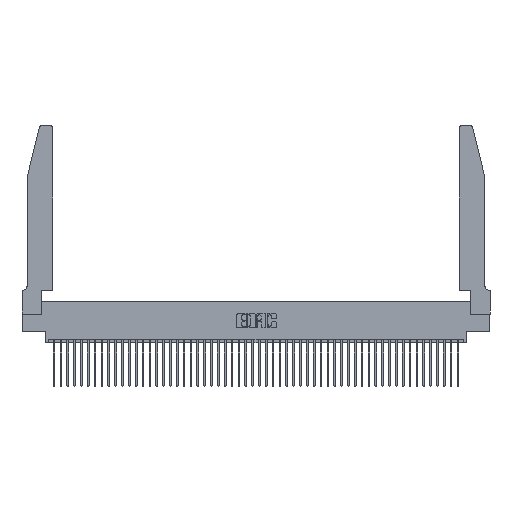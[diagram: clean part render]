
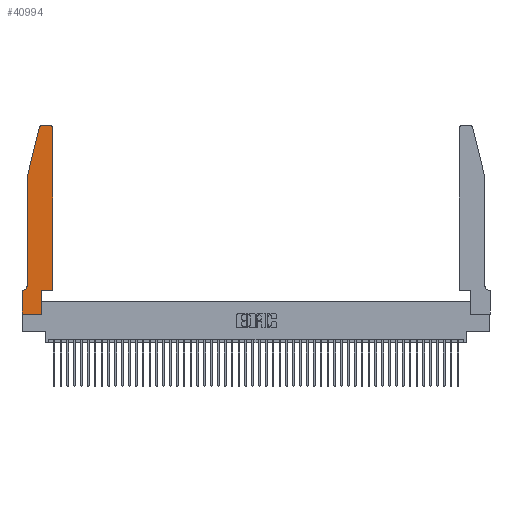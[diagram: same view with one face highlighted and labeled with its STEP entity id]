
A CAD part, top view. The second image highlights one B-rep face of the part: STEP entity #40994.
In plain terms, the highlighted planar face has unit normal (0, 0, 1).
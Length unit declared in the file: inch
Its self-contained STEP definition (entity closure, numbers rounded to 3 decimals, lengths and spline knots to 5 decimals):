
#375 = VERTEX_POINT ( 'NONE', #23162 ) ;
#771 = VERTEX_POINT ( 'NONE', #3307 ) ;
#784 = DIRECTION ( 'NONE',  ( 1., 0., 0. ) ) ;
#2011 = LINE ( 'NONE', #36926, #9230 ) ;
#2113 = VECTOR ( 'NONE', #45506, 39.37008 ) ;
#2149 = EDGE_CURVE ( 'NONE', #18100, #37735, #42309, .T. ) ;
#2790 = DIRECTION ( 'NONE',  ( 0., 0., 1. ) ) ;
#2897 = EDGE_CURVE ( 'NONE', #375, #42579, #21915, .T. ) ;
#3307 = CARTESIAN_POINT ( 'NONE',  ( 0.4505, 0.35, 0.37 ) ) ;
#3364 = ORIENTED_EDGE ( 'NONE', *, *, #41701, .T. ) ;
#5759 = EDGE_CURVE ( 'NONE', #32622, #375, #25288, .T. ) ;
#6160 = VECTOR ( 'NONE', #47278, 39.37008 ) ;
#6605 = ORIENTED_EDGE ( 'NONE', *, *, #2149, .T. ) ;
#6649 = DIRECTION ( 'NONE',  ( 1., 0., 0. ) ) ;
#7115 = AXIS2_PLACEMENT_3D ( 'NONE', #40677, #36499, #13609 ) ;
#7495 = LINE ( 'NONE', #33972, #2113 ) ;
#8352 = DIRECTION ( 'NONE',  ( 0., -1., 0. ) ) ;
#8482 = EDGE_CURVE ( 'NONE', #42579, #31190, #42761, .T. ) ;
#8602 = CARTESIAN_POINT ( 'NONE',  ( 0.2865, 0., 0.37 ) ) ;
#9230 = VECTOR ( 'NONE', #33563, 39.37008 ) ;
#10629 = EDGE_CURVE ( 'NONE', #37735, #46674, #25936, .T. ) ;
#10841 = EDGE_CURVE ( 'NONE', #18579, #32622, #27144, .T. ) ;
#11779 = ORIENTED_EDGE ( 'NONE', *, *, #10841, .T. ) ;
#12207 = DIRECTION ( 'NONE',  ( 0., 0., 1. ) ) ;
#12232 = CARTESIAN_POINT ( 'NONE',  ( 0., 0., 0.37 ) ) ;
#13609 = DIRECTION ( 'NONE',  ( 1., 0., 0. ) ) ;
#14402 = CARTESIAN_POINT ( 'NONE',  ( 0.0755, 2., 0.37 ) ) ;
#14742 = DIRECTION ( 'NONE',  ( -1., 0., 0. ) ) ;
#14904 = CARTESIAN_POINT ( 'NONE',  ( 0.0755, 0.35, 0.37 ) ) ;
#15730 = CARTESIAN_POINT ( 'NONE',  ( 0.0755, 2., 0.37 ) ) ;
#16501 = CARTESIAN_POINT ( 'NONE',  ( 0., 0.35, 0.37 ) ) ;
#17011 = ORIENTED_EDGE ( 'NONE', *, *, #10629, .T. ) ;
#17167 = EDGE_CURVE ( 'NONE', #771, #18100, #24721, .T. ) ;
#17384 = LINE ( 'NONE', #26004, #25172 ) ;
#18100 = VERTEX_POINT ( 'NONE', #32511 ) ;
#18579 = VERTEX_POINT ( 'NONE', #35409 ) ;
#19600 = EDGE_CURVE ( 'NONE', #31190, #21542, #17384, .T. ) ;
#20029 = CARTESIAN_POINT ( 'NONE',  ( 0.2865, 0.35, 0.37 ) ) ;
#20559 = CARTESIAN_POINT ( 'NONE',  ( 0.4505, 0.35, 0.37 ) ) ;
#20562 = ORIENTED_EDGE ( 'NONE', *, *, #17167, .T. ) ;
#20934 = CARTESIAN_POINT ( 'NONE',  ( 0.2605, 2.75, 0.37 ) ) ;
#20989 = VERTEX_POINT ( 'NONE', #20029 ) ;
#21318 = AXIS2_PLACEMENT_3D ( 'NONE', #44787, #2790, #6649 ) ;
#21542 = VERTEX_POINT ( 'NONE', #12232 ) ;
#21915 = CIRCLE ( 'NONE', #22912, 0.07 ) ;
#22912 = AXIS2_PLACEMENT_3D ( 'NONE', #36010, #40499, #31117 ) ;
#23162 = CARTESIAN_POINT ( 'NONE',  ( 0.0755, 0.42, 0.37 ) ) ;
#24636 = EDGE_LOOP ( 'NONE', ( #17011, #3364, #11779, #31216, #34643, #43755, #44203, #46349, #46290, #40302, #20562, #6605 ) ) ;
#24721 = LINE ( 'NONE', #20559, #6160 ) ;
#25172 = VECTOR ( 'NONE', #30637, 39.37008 ) ;
#25288 = LINE ( 'NONE', #15730, #45593 ) ;
#25636 = DIRECTION ( 'NONE',  ( -0.239, -0.971, 0. ) ) ;
#25936 = LINE ( 'NONE', #20934, #31255 ) ;
#26004 = CARTESIAN_POINT ( 'NONE',  ( 0., 0., 0.37 ) ) ;
#27144 = LINE ( 'NONE', #14402, #33655 ) ;
#28361 = LINE ( 'NONE', #39063, #40288 ) ;
#30637 = DIRECTION ( 'NONE',  ( 0., -1., 0. ) ) ;
#30808 = CARTESIAN_POINT ( 'NONE',  ( 0.284, 2.75, 0.37 ) ) ;
#31117 = DIRECTION ( 'NONE',  ( -1., 0., 0. ) ) ;
#31190 = VERTEX_POINT ( 'NONE', #16501 ) ;
#31216 = ORIENTED_EDGE ( 'NONE', *, *, #5759, .T. ) ;
#31255 = VECTOR ( 'NONE', #47661, 39.37008 ) ;
#31636 = CARTESIAN_POINT ( 'NONE',  ( 0.0055, 0.35, 0.37 ) ) ;
#31697 = DIRECTION ( 'NONE',  ( 1., 0., 0. ) ) ;
#32511 = CARTESIAN_POINT ( 'NONE',  ( 0.4505, 2.72, 0.37 ) ) ;
#32622 = VERTEX_POINT ( 'NONE', #48794 ) ;
#33563 = DIRECTION ( 'NONE',  ( 0., 1., 0. ) ) ;
#33655 = VECTOR ( 'NONE', #25636, 39.37008 ) ;
#33972 = CARTESIAN_POINT ( 'NONE',  ( 0.4505, 0.35, 0.37 ) ) ;
#34060 = EDGE_CURVE ( 'NONE', #21542, #49346, #28361, .T. ) ;
#34562 = CIRCLE ( 'NONE', #21318, 0.03 ) ;
#34643 = ORIENTED_EDGE ( 'NONE', *, *, #2897, .T. ) ;
#35409 = CARTESIAN_POINT ( 'NONE',  ( 0.25487, 2.72718, 0.37 ) ) ;
#36010 = CARTESIAN_POINT ( 'NONE',  ( 0.0055, 0.42, 0.37 ) ) ;
#36499 = DIRECTION ( 'NONE',  ( 0., 0., 1. ) ) ;
#36819 = VECTOR ( 'NONE', #14742, 39.37008 ) ;
#36926 = CARTESIAN_POINT ( 'NONE',  ( 0.2865, 0.35, 0.37 ) ) ;
#37735 = VERTEX_POINT ( 'NONE', #45632 ) ;
#38616 = CARTESIAN_POINT ( 'NONE',  ( 0.4205, 2.72, 0.37 ) ) ;
#39063 = CARTESIAN_POINT ( 'NONE',  ( 0., 0., 0.37 ) ) ;
#39844 = AXIS2_PLACEMENT_3D ( 'NONE', #38616, #12207, #784 ) ;
#40288 = VECTOR ( 'NONE', #31697, 39.37008 ) ;
#40302 = ORIENTED_EDGE ( 'NONE', *, *, #43199, .T. ) ;
#40499 = DIRECTION ( 'NONE',  ( 0., 0., -1. ) ) ;
#40677 = CARTESIAN_POINT ( 'NONE',  ( 0., 0.35, 0.37 ) ) ;
#40994 = ADVANCED_FACE ( 'NONE', ( #45415 ), #48201, .T. ) ;
#41701 = EDGE_CURVE ( 'NONE', #46674, #18579, #34562, .T. ) ;
#42309 = CIRCLE ( 'NONE', #39844, 0.03 ) ;
#42579 = VERTEX_POINT ( 'NONE', #31636 ) ;
#42761 = LINE ( 'NONE', #14904, #36819 ) ;
#43199 = EDGE_CURVE ( 'NONE', #20989, #771, #7495, .T. ) ;
#43755 = ORIENTED_EDGE ( 'NONE', *, *, #8482, .T. ) ;
#43840 = EDGE_CURVE ( 'NONE', #49346, #20989, #2011, .T. ) ;
#44203 = ORIENTED_EDGE ( 'NONE', *, *, #19600, .T. ) ;
#44787 = CARTESIAN_POINT ( 'NONE',  ( 0.284, 2.72, 0.37 ) ) ;
#45415 = FACE_OUTER_BOUND ( 'NONE', #24636, .T. ) ;
#45506 = DIRECTION ( 'NONE',  ( 1., 0., 0. ) ) ;
#45593 = VECTOR ( 'NONE', #8352, 39.37008 ) ;
#45632 = CARTESIAN_POINT ( 'NONE',  ( 0.4205, 2.75, 0.37 ) ) ;
#46290 = ORIENTED_EDGE ( 'NONE', *, *, #43840, .T. ) ;
#46349 = ORIENTED_EDGE ( 'NONE', *, *, #34060, .T. ) ;
#46674 = VERTEX_POINT ( 'NONE', #30808 ) ;
#47278 = DIRECTION ( 'NONE',  ( 0., 1., 0. ) ) ;
#47661 = DIRECTION ( 'NONE',  ( -1., 0., 0. ) ) ;
#48201 = PLANE ( 'NONE',  #7115 ) ;
#48794 = CARTESIAN_POINT ( 'NONE',  ( 0.0755, 2., 0.37 ) ) ;
#49346 = VERTEX_POINT ( 'NONE', #8602 ) ;
